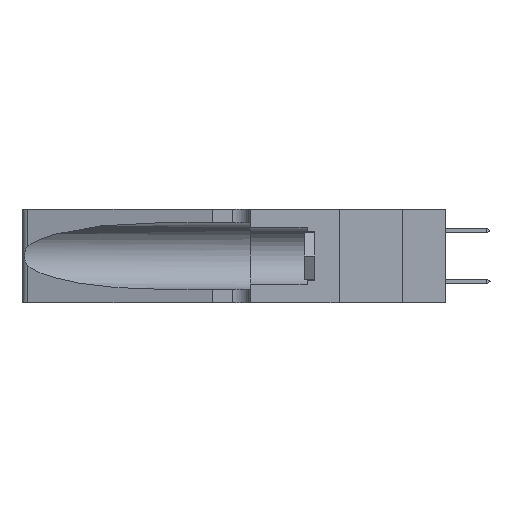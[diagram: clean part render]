
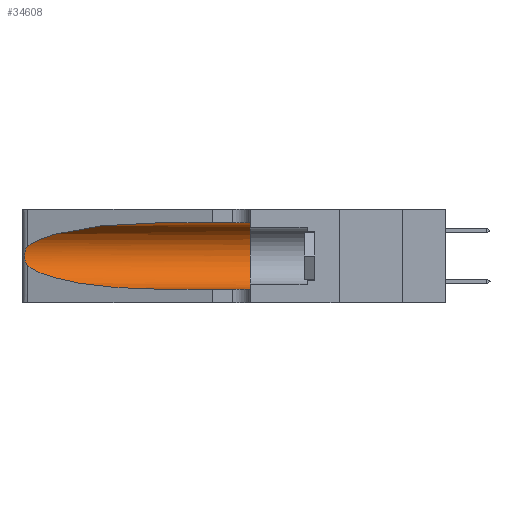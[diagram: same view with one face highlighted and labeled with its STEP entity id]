
A CAD part, left-side view. The second image highlights one B-rep face of the part: STEP entity #34608.
In plain terms, the highlighted cylindrical face has radius 3.308 mm (diameter 6.617 mm), a partial arc.
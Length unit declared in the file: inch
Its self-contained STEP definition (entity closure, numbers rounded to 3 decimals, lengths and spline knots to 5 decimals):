
#269 = CARTESIAN_POINT ( 'NONE',  ( 0.25487, 1.22718, 0.22369 ) ) ;
#2241 = EDGE_CURVE ( 'NONE', #22407, #10159, #21526, .T. ) ;
#2275 = EDGE_CURVE ( 'NONE', #18230, #25839, #10684, .T. ) ;
#2398 = CARTESIAN_POINT ( 'NONE',  ( 0.25487, 1.22718, 0.14631 ) ) ;
#2514 = CARTESIAN_POINT ( 'NONE',  ( 0.25789, 1.23486, 0.15765 ) ) ;
#2781 = DIRECTION ( 'NONE',  ( 0., -1., 0. ) ) ;
#2960 = ORIENTED_EDGE ( 'NONE', *, *, #17632, .F. ) ;
#3453 =( BOUNDED_CURVE ( )  B_SPLINE_CURVE ( 3, ( #2398, #36376, #22357, #5390 ),
 .UNSPECIFIED., .F., .F. ) 
 B_SPLINE_CURVE_WITH_KNOTS ( ( 4, 4 ),
 ( 3.44316, 4.71239 ),
 .UNSPECIFIED. ) 
 CURVE ( )  GEOMETRIC_REPRESENTATION_ITEM ( )  RATIONAL_B_SPLINE_CURVE ( ( 1., 0.87, 0.87, 1. ) ) 
 REPRESENTATION_ITEM ( '' )  );
#4686 = CIRCLE ( 'NONE', #22798, 0.13025 ) ;
#5107 = AXIS2_PLACEMENT_3D ( 'NONE', #14056, #28036, #16890 ) ;
#5265 = CARTESIAN_POINT ( 'NONE',  ( 0.25555, 1.22994, 0.2215 ) ) ;
#5379 = CARTESIAN_POINT ( 'NONE',  ( 0.25555, 1.22993, 0.14849 ) ) ;
#5390 = CARTESIAN_POINT ( 'NONE',  ( 0.1305, 0.72297, 0.05475 ) ) ;
#5955 = ORIENTED_EDGE ( 'NONE', *, *, #14383, .F. ) ;
#6502 = CARTESIAN_POINT ( 'NONE',  ( 0.25487, 1.22718, 0.14631 ) ) ;
#6939 = CARTESIAN_POINT ( 'NONE',  ( 0.1305, 0.72297, 0.31525 ) ) ;
#7391 = CARTESIAN_POINT ( 'NONE',  ( 0.1305, 0.35, 0.185 ) ) ;
#8134 = CARTESIAN_POINT ( 'NONE',  ( 0.25487, 1.22718, 0.22369 ) ) ;
#8340 = ORIENTED_EDGE ( 'NONE', *, *, #30781, .T. ) ;
#9002 =( BOUNDED_CURVE ( )  B_SPLINE_CURVE ( 3, ( #6939, #23881, #9785, #29566 ),
 .UNSPECIFIED., .F., .T. ) 
 B_SPLINE_CURVE_WITH_KNOTS ( ( 4, 4 ),
 ( 1.5708, 2.84003 ),
 .UNSPECIFIED. ) 
 CURVE ( )  GEOMETRIC_REPRESENTATION_ITEM ( )  RATIONAL_B_SPLINE_CURVE ( ( 1., 0.87, 0.87, 1. ) ) 
 REPRESENTATION_ITEM ( '' )  );
#9785 = CARTESIAN_POINT ( 'NONE',  ( 0.2373, 1.15595, 0.28018 ) ) ;
#10159 = VERTEX_POINT ( 'NONE', #6502 ) ;
#10246 = DIRECTION ( 'NONE',  ( 0., 0., 1. ) ) ;
#10684 = LINE ( 'NONE', #12035, #26579 ) ;
#10976 = CARTESIAN_POINT ( 'NONE',  ( 0.25787, 1.23484, 0.2124 ) ) ;
#11518 = CARTESIAN_POINT ( 'NONE',  ( 0.1305, 1.61858, 0.31525 ) ) ;
#12035 = CARTESIAN_POINT ( 'NONE',  ( 0.1305, 1.61858, 0.05475 ) ) ;
#13808 = CARTESIAN_POINT ( 'NONE',  ( 0.26018, 1.23835, 0.19895 ) ) ;
#14056 = CARTESIAN_POINT ( 'NONE',  ( 0.1305, 1.61858, 0.185 ) ) ;
#14383 = EDGE_CURVE ( 'NONE', #28387, #23461, #33025, .T. ) ;
#16647 = CARTESIAN_POINT ( 'NONE',  ( 0.26075, 1.23896, 0.178 ) ) ;
#16890 = DIRECTION ( 'NONE',  ( 0., 0., -1. ) ) ;
#17218 = CARTESIAN_POINT ( 'NONE',  ( 0.1305, 0.72297, 0.05475 ) ) ;
#17365 = CARTESIAN_POINT ( 'NONE',  ( 0.1305, 0.35, 0.05475 ) ) ;
#17632 = EDGE_CURVE ( 'NONE', #23461, #25839, #4686, .T. ) ;
#17985 = VECTOR ( 'NONE', #19825, 39.37008 ) ;
#18230 = VERTEX_POINT ( 'NONE', #17218 ) ;
#19048 = EDGE_CURVE ( 'NONE', #28387, #22407, #9002, .T. ) ;
#19496 = CARTESIAN_POINT ( 'NONE',  ( 0.25856, 1.23593, 0.16098 ) ) ;
#19825 = DIRECTION ( 'NONE',  ( 0., -1., 0. ) ) ;
#20153 = CYLINDRICAL_SURFACE ( 'NONE', #5107, 0.13025 ) ;
#21526 = B_SPLINE_CURVE_WITH_KNOTS ( 'NONE', 3,
 ( #8134, #5265, #22218, #10976, #30748, #13808, #33570, #16647, #36366, #19496, #2514, #22344, #5379, #25195 ),
 .UNSPECIFIED., .F., .F.,
 ( 4, 2, 2, 2, 2, 2, 4 ),
 ( 0., 0.00027, 0.00053, 0.00107, 0.0016, 0.00187, 0.00214 ),
 .UNSPECIFIED. ) ;
#22218 = CARTESIAN_POINT ( 'NONE',  ( 0.25639, 1.23184, 0.21858 ) ) ;
#22344 = CARTESIAN_POINT ( 'NONE',  ( 0.25639, 1.23186, 0.15144 ) ) ;
#22357 = CARTESIAN_POINT ( 'NONE',  ( 0.18966, 0.96281, 0.05475 ) ) ;
#22407 = VERTEX_POINT ( 'NONE', #269 ) ;
#22798 = AXIS2_PLACEMENT_3D ( 'NONE', #7391, #27160, #10246 ) ;
#23461 = VERTEX_POINT ( 'NONE', #30494 ) ;
#23881 = CARTESIAN_POINT ( 'NONE',  ( 0.18966, 0.96281, 0.31525 ) ) ;
#25195 = CARTESIAN_POINT ( 'NONE',  ( 0.25487, 1.22718, 0.14631 ) ) ;
#25839 = VERTEX_POINT ( 'NONE', #17365 ) ;
#26046 = EDGE_LOOP ( 'NONE', ( #30371, #34466, #8340, #30644, #2960, #5955 ) ) ;
#26579 = VECTOR ( 'NONE', #2781, 39.37008 ) ;
#27160 = DIRECTION ( 'NONE',  ( 0., 1., 0. ) ) ;
#28036 = DIRECTION ( 'NONE',  ( 0., -1., 0. ) ) ;
#28387 = VERTEX_POINT ( 'NONE', #35791 ) ;
#29566 = CARTESIAN_POINT ( 'NONE',  ( 0.25487, 1.22718, 0.22369 ) ) ;
#30169 = FACE_OUTER_BOUND ( 'NONE', #26046, .T. ) ;
#30371 = ORIENTED_EDGE ( 'NONE', *, *, #19048, .T. ) ;
#30494 = CARTESIAN_POINT ( 'NONE',  ( 0.1305, 0.35, 0.31525 ) ) ;
#30644 = ORIENTED_EDGE ( 'NONE', *, *, #2275, .T. ) ;
#30748 = CARTESIAN_POINT ( 'NONE',  ( 0.25854, 1.2359, 0.20912 ) ) ;
#30781 = EDGE_CURVE ( 'NONE', #10159, #18230, #3453, .T. ) ;
#33025 = LINE ( 'NONE', #11518, #17985 ) ;
#33570 = CARTESIAN_POINT ( 'NONE',  ( 0.26075, 1.23896, 0.19203 ) ) ;
#34466 = ORIENTED_EDGE ( 'NONE', *, *, #2241, .T. ) ;
#34608 = ADVANCED_FACE ( 'NONE', ( #30169 ), #20153, .F. ) ;
#35791 = CARTESIAN_POINT ( 'NONE',  ( 0.1305, 0.72297, 0.31525 ) ) ;
#36366 = CARTESIAN_POINT ( 'NONE',  ( 0.26017, 1.23833, 0.17102 ) ) ;
#36376 = CARTESIAN_POINT ( 'NONE',  ( 0.2373, 1.15595, 0.08982 ) ) ;
